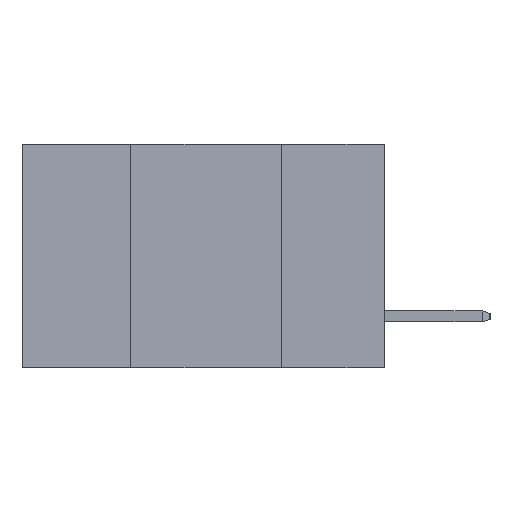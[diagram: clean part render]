
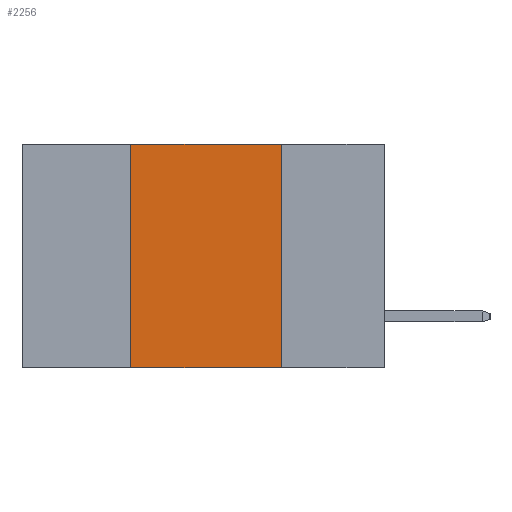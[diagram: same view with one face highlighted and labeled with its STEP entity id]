
A CAD part, left-side view. The second image highlights one B-rep face of the part: STEP entity #2256.
In plain terms, the highlighted planar face has unit normal (-1, 0, 0).
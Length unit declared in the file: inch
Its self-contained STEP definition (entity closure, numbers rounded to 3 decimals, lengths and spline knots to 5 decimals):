
#300 = VERTEX_POINT ( 'NONE', #11436 ) ;
#548 = EDGE_CURVE ( 'NONE', #15267, #3177, #14922, .T. ) ;
#805 = CARTESIAN_POINT ( 'NONE',  ( 0., 0.17, -0.37 ) ) ;
#1516 = EDGE_CURVE ( 'NONE', #300, #15804, #13190, .T. ) ;
#2040 = VECTOR ( 'NONE', #5519, 39.37008 ) ;
#2256 = ADVANCED_FACE ( 'NONE', ( #8814 ), #9623, .F. ) ;
#2357 = CARTESIAN_POINT ( 'NONE',  ( 0., 0.42, 0. ) ) ;
#2767 = LINE ( 'NONE', #6564, #13451 ) ;
#3177 = VERTEX_POINT ( 'NONE', #5467 ) ;
#3645 = ORIENTED_EDGE ( 'NONE', *, *, #548, .F. ) ;
#3832 = VECTOR ( 'NONE', #14191, 39.37008 ) ;
#4216 = EDGE_CURVE ( 'NONE', #3177, #300, #13054, .T. ) ;
#5032 = CARTESIAN_POINT ( 'NONE',  ( 0., 0.6, 0. ) ) ;
#5076 = DIRECTION ( 'NONE',  ( 1., 0., 0. ) ) ;
#5467 = CARTESIAN_POINT ( 'NONE',  ( 0., 0.42, 0. ) ) ;
#5519 = DIRECTION ( 'NONE',  ( 0., 0., -1. ) ) ;
#6060 = VECTOR ( 'NONE', #14623, 39.37008 ) ;
#6564 = CARTESIAN_POINT ( 'NONE',  ( 0., 0.6, -0.37 ) ) ;
#7259 = EDGE_LOOP ( 'NONE', ( #13913, #10729, #3645, #7838 ) ) ;
#7735 = CARTESIAN_POINT ( 'NONE',  ( 0., 0.6, 0. ) ) ;
#7838 = ORIENTED_EDGE ( 'NONE', *, *, #17552, .T. ) ;
#8303 = CARTESIAN_POINT ( 'NONE',  ( 0., 0.42, -0.37 ) ) ;
#8814 = FACE_OUTER_BOUND ( 'NONE', #7259, .T. ) ;
#9099 = CARTESIAN_POINT ( 'NONE',  ( 0., 0.17, 0. ) ) ;
#9623 = PLANE ( 'NONE',  #15291 ) ;
#10729 = ORIENTED_EDGE ( 'NONE', *, *, #4216, .F. ) ;
#11436 = CARTESIAN_POINT ( 'NONE',  ( 0., 0.17, 0. ) ) ;
#13054 = LINE ( 'NONE', #7735, #6060 ) ;
#13190 = LINE ( 'NONE', #9099, #2040 ) ;
#13451 = VECTOR ( 'NONE', #17486, 39.37008 ) ;
#13913 = ORIENTED_EDGE ( 'NONE', *, *, #1516, .F. ) ;
#14191 = DIRECTION ( 'NONE',  ( 0., 0., 1. ) ) ;
#14328 = DIRECTION ( 'NONE',  ( 0., 0., -1. ) ) ;
#14623 = DIRECTION ( 'NONE',  ( 0., -1., 0. ) ) ;
#14922 = LINE ( 'NONE', #2357, #3832 ) ;
#15267 = VERTEX_POINT ( 'NONE', #8303 ) ;
#15291 = AXIS2_PLACEMENT_3D ( 'NONE', #5032, #5076, #14328 ) ;
#15804 = VERTEX_POINT ( 'NONE', #805 ) ;
#17486 = DIRECTION ( 'NONE',  ( 0., -1., 0. ) ) ;
#17552 = EDGE_CURVE ( 'NONE', #15267, #15804, #2767, .T. ) ;
